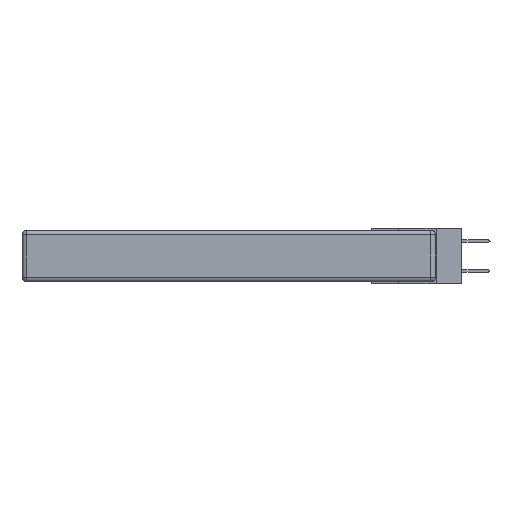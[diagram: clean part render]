
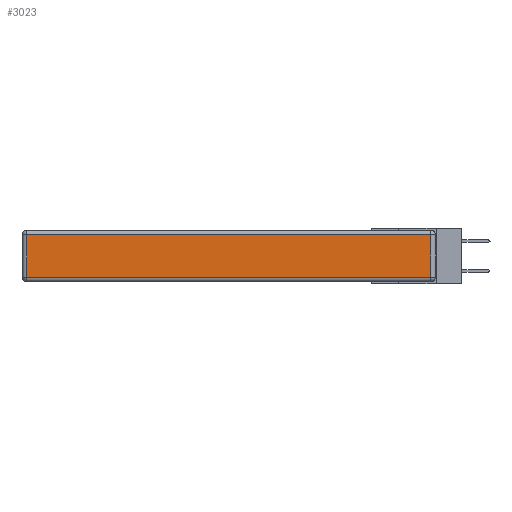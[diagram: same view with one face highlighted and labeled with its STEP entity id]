
A CAD part, left-side view. The second image highlights one B-rep face of the part: STEP entity #3023.
In plain terms, the highlighted planar face has unit normal (-1, 0, 0).
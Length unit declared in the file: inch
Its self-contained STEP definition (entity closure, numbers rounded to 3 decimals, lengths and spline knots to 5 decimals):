
#3023 = ADVANCED_FACE ( 'NONE', ( #16449 ), #22351, .T. ) ;
#3563 = VERTEX_POINT ( 'NONE', #30002 ) ;
#4305 = EDGE_CURVE ( 'NONE', #8125, #3563, #15133, .T. ) ;
#4317 = ORIENTED_EDGE ( 'NONE', *, *, #25406, .T. ) ;
#4590 = DIRECTION ( 'NONE',  ( 0., 0., 1. ) ) ;
#5079 = VECTOR ( 'NONE', #11912, 39.37008 ) ;
#5742 = VERTEX_POINT ( 'NONE', #14887 ) ;
#7344 = VECTOR ( 'NONE', #27199, 39.37008 ) ;
#7436 = LINE ( 'NONE', #14700, #31724 ) ;
#8025 = CARTESIAN_POINT ( 'NONE',  ( 0., 2.72, -0.03 ) ) ;
#8125 = VERTEX_POINT ( 'NONE', #11396 ) ;
#8935 = VERTEX_POINT ( 'NONE', #8025 ) ;
#9380 = AXIS2_PLACEMENT_3D ( 'NONE', #11889, #19498, #4590 ) ;
#9634 = ORIENTED_EDGE ( 'NONE', *, *, #14669, .T. ) ;
#10223 = ORIENTED_EDGE ( 'NONE', *, *, #4305, .T. ) ;
#10443 = DIRECTION ( 'NONE',  ( 0., 0., -1. ) ) ;
#10505 = VECTOR ( 'NONE', #10443, 39.37008 ) ;
#11396 = CARTESIAN_POINT ( 'NONE',  ( 0., 2.72, -0.313 ) ) ;
#11889 = CARTESIAN_POINT ( 'NONE',  ( 0., 0., -0.343 ) ) ;
#11912 = DIRECTION ( 'NONE',  ( 0., -1., 0. ) ) ;
#14102 = LINE ( 'NONE', #28443, #10505 ) ;
#14391 = CARTESIAN_POINT ( 'NONE',  ( 0., 0., -0.313 ) ) ;
#14669 = EDGE_CURVE ( 'NONE', #3563, #5742, #7436, .T. ) ;
#14700 = CARTESIAN_POINT ( 'NONE',  ( 0., 0.03, -0.343 ) ) ;
#14887 = CARTESIAN_POINT ( 'NONE',  ( 0., 0.03, -0.03 ) ) ;
#15133 = LINE ( 'NONE', #14391, #5079 ) ;
#16293 = ORIENTED_EDGE ( 'NONE', *, *, #32797, .T. ) ;
#16449 = FACE_OUTER_BOUND ( 'NONE', #31465, .T. ) ;
#19350 = CARTESIAN_POINT ( 'NONE',  ( 0., 2.75, -0.03 ) ) ;
#19498 = DIRECTION ( 'NONE',  ( -1., 0., 0. ) ) ;
#22351 = PLANE ( 'NONE',  #9380 ) ;
#25406 = EDGE_CURVE ( 'NONE', #8935, #8125, #14102, .T. ) ;
#25668 = DIRECTION ( 'NONE',  ( 0., 0., 1. ) ) ;
#27199 = DIRECTION ( 'NONE',  ( 0., 1., 0. ) ) ;
#28042 = LINE ( 'NONE', #19350, #7344 ) ;
#28443 = CARTESIAN_POINT ( 'NONE',  ( 0., 2.72, -0.343 ) ) ;
#30002 = CARTESIAN_POINT ( 'NONE',  ( 0., 0.03, -0.313 ) ) ;
#31465 = EDGE_LOOP ( 'NONE', ( #10223, #9634, #16293, #4317 ) ) ;
#31724 = VECTOR ( 'NONE', #25668, 39.37008 ) ;
#32797 = EDGE_CURVE ( 'NONE', #5742, #8935, #28042, .T. ) ;
